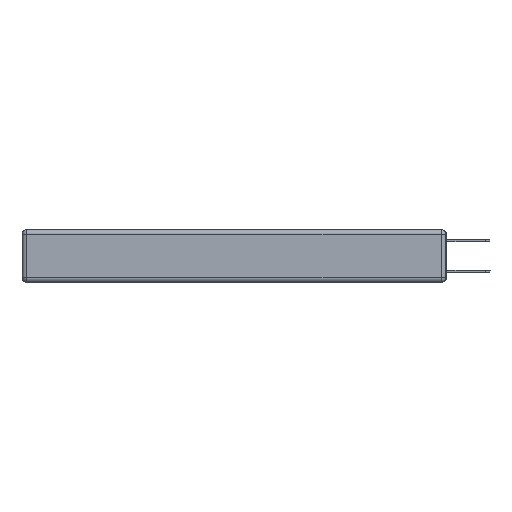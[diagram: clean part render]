
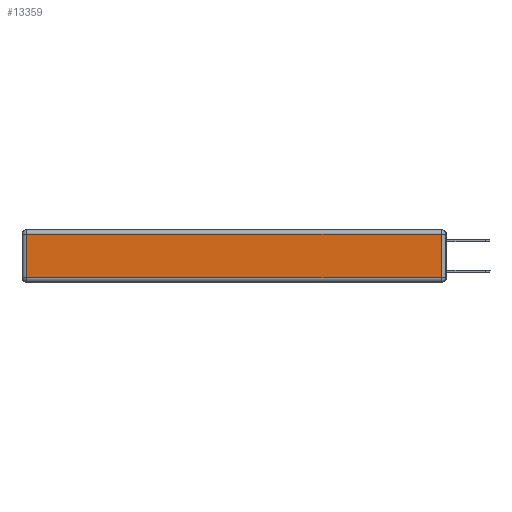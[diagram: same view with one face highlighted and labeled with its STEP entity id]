
A CAD part, left-side view. The second image highlights one B-rep face of the part: STEP entity #13359.
In plain terms, the highlighted planar face has unit normal (-1, 0, 0).
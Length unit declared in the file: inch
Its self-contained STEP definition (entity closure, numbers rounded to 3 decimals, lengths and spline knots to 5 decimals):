
#1227 = VECTOR ( 'NONE', #16063, 39.37008 ) ;
#1843 = CARTESIAN_POINT ( 'NONE',  ( 0., 0.03, -0.343 ) ) ;
#2104 = CARTESIAN_POINT ( 'NONE',  ( 0., 2.72, -0.313 ) ) ;
#2907 = CARTESIAN_POINT ( 'NONE',  ( 0., 2.75, -0.03 ) ) ;
#3186 = CARTESIAN_POINT ( 'NONE',  ( 0., 2.72, -0.343 ) ) ;
#3278 = DIRECTION ( 'NONE',  ( 0., 0., 1. ) ) ;
#3856 = VECTOR ( 'NONE', #7184, 39.37008 ) ;
#3996 = EDGE_CURVE ( 'NONE', #11198, #7098, #12254, .T. ) ;
#4003 = EDGE_CURVE ( 'NONE', #6510, #11198, #7758, .T. ) ;
#4346 = AXIS2_PLACEMENT_3D ( 'NONE', #14532, #7478, #11823 ) ;
#4531 = CARTESIAN_POINT ( 'NONE',  ( 0., 2.72, -0.03 ) ) ;
#5221 = LINE ( 'NONE', #3186, #12452 ) ;
#5928 = FACE_OUTER_BOUND ( 'NONE', #6210, .T. ) ;
#6210 = EDGE_LOOP ( 'NONE', ( #14853, #15181, #16952, #8842 ) ) ;
#6510 = VERTEX_POINT ( 'NONE', #2104 ) ;
#7098 = VERTEX_POINT ( 'NONE', #13181 ) ;
#7184 = DIRECTION ( 'NONE',  ( 0., 1., 0. ) ) ;
#7478 = DIRECTION ( 'NONE',  ( -1., 0., 0. ) ) ;
#7758 = LINE ( 'NONE', #10531, #1227 ) ;
#8442 = PLANE ( 'NONE',  #4346 ) ;
#8842 = ORIENTED_EDGE ( 'NONE', *, *, #16382, .T. ) ;
#9256 = LINE ( 'NONE', #2907, #3856 ) ;
#9997 = CARTESIAN_POINT ( 'NONE',  ( 0., 0.03, -0.313 ) ) ;
#10315 = VERTEX_POINT ( 'NONE', #4531 ) ;
#10531 = CARTESIAN_POINT ( 'NONE',  ( 0., 0., -0.313 ) ) ;
#11198 = VERTEX_POINT ( 'NONE', #9997 ) ;
#11823 = DIRECTION ( 'NONE',  ( 0., 0., 1. ) ) ;
#12043 = VECTOR ( 'NONE', #3278, 39.37008 ) ;
#12125 = DIRECTION ( 'NONE',  ( 0., 0., -1. ) ) ;
#12254 = LINE ( 'NONE', #1843, #12043 ) ;
#12452 = VECTOR ( 'NONE', #12125, 39.37008 ) ;
#13181 = CARTESIAN_POINT ( 'NONE',  ( 0., 0.03, -0.03 ) ) ;
#13359 = ADVANCED_FACE ( 'NONE', ( #5928 ), #8442, .T. ) ;
#14532 = CARTESIAN_POINT ( 'NONE',  ( 0., 0., -0.343 ) ) ;
#14853 = ORIENTED_EDGE ( 'NONE', *, *, #4003, .T. ) ;
#15181 = ORIENTED_EDGE ( 'NONE', *, *, #3996, .T. ) ;
#16063 = DIRECTION ( 'NONE',  ( 0., -1., 0. ) ) ;
#16382 = EDGE_CURVE ( 'NONE', #10315, #6510, #5221, .T. ) ;
#16921 = EDGE_CURVE ( 'NONE', #7098, #10315, #9256, .T. ) ;
#16952 = ORIENTED_EDGE ( 'NONE', *, *, #16921, .T. ) ;
